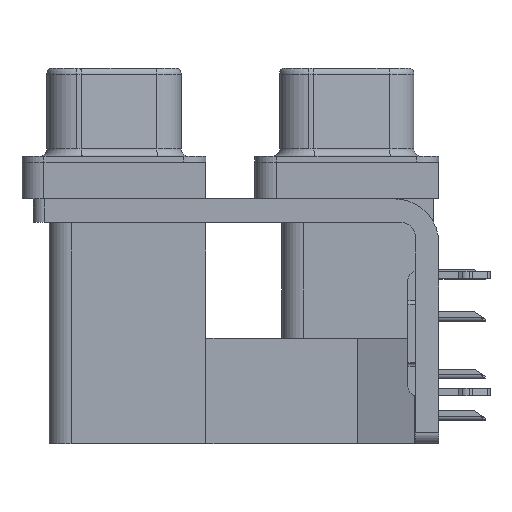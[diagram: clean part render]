
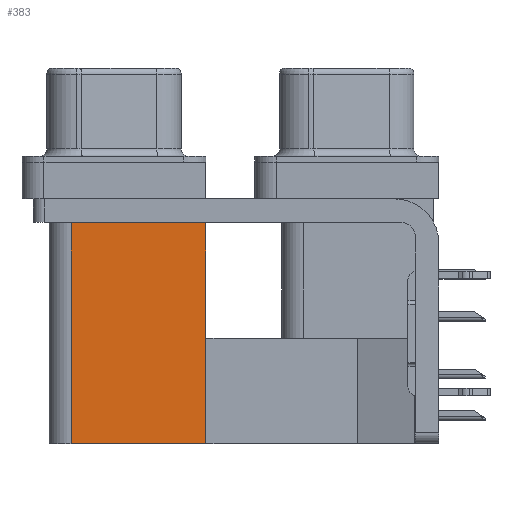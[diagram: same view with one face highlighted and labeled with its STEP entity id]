
A CAD part, left-side view. The second image highlights one B-rep face of the part: STEP entity #383.
In plain terms, the highlighted planar face has unit normal (-1, 0, 0).
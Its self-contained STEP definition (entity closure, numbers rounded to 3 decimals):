
#65 = AXIS2_PLACEMENT_3D ( 'NONE', #16014, #2208, #369 ) ;
#312 = VERTEX_POINT ( 'NONE', #13531 ) ;
#369 = DIRECTION ( 'NONE',  ( 0., 0., -1. ) ) ;
#383 = ADVANCED_FACE ( 'NONE', ( #8005 ), #22569, .F. ) ;
#1462 = LINE ( 'NONE', #24841, #5147 ) ;
#1758 = VECTOR ( 'NONE', #3354, 1000. ) ;
#1886 = EDGE_CURVE ( 'NONE', #18870, #14681, #2831, .T. ) ;
#2208 = DIRECTION ( 'NONE',  ( 1., 0., 0. ) ) ;
#2485 = VECTOR ( 'NONE', #20062, 1000. ) ;
#2831 = LINE ( 'NONE', #25289, #1758 ) ;
#3354 = DIRECTION ( 'NONE',  ( 0., 0., 1. ) ) ;
#4014 = ORIENTED_EDGE ( 'NONE', *, *, #1886, .T. ) ;
#4415 = EDGE_CURVE ( 'NONE', #18870, #7563, #24840, .T. ) ;
#5147 = VECTOR ( 'NONE', #17344, 1000. ) ;
#6847 = CARTESIAN_POINT ( 'NONE',  ( 3.79, 9.6, -19.2 ) ) ;
#7563 = VERTEX_POINT ( 'NONE', #13331 ) ;
#7720 = ORIENTED_EDGE ( 'NONE', *, *, #4415, .F. ) ;
#8005 = FACE_OUTER_BOUND ( 'NONE', #17991, .T. ) ;
#10920 = CARTESIAN_POINT ( 'NONE',  ( 3.79, 9.6, -2.5 ) ) ;
#11751 = ORIENTED_EDGE ( 'NONE', *, *, #19619, .T. ) ;
#13331 = CARTESIAN_POINT ( 'NONE',  ( 3.79, 18.8, -19.2 ) ) ;
#13531 = CARTESIAN_POINT ( 'NONE',  ( 3.79, 18.8, -2.5 ) ) ;
#14681 = VERTEX_POINT ( 'NONE', #10920 ) ;
#15312 = VECTOR ( 'NONE', #16956, 1000. ) ;
#16014 = CARTESIAN_POINT ( 'NONE',  ( 3.79, 9.6, -19.2 ) ) ;
#16956 = DIRECTION ( 'NONE',  ( 0., 1., 0. ) ) ;
#17344 = DIRECTION ( 'NONE',  ( 0., 0., 1. ) ) ;
#17991 = EDGE_LOOP ( 'NONE', ( #11751, #24680, #7720, #4014 ) ) ;
#18088 = CARTESIAN_POINT ( 'NONE',  ( 3.79, 9.6, -2.5 ) ) ;
#18870 = VERTEX_POINT ( 'NONE', #24719 ) ;
#19619 = EDGE_CURVE ( 'NONE', #14681, #312, #19804, .T. ) ;
#19804 = LINE ( 'NONE', #18088, #2485 ) ;
#20062 = DIRECTION ( 'NONE',  ( 0., 1., 0. ) ) ;
#22569 = PLANE ( 'NONE',  #65 ) ;
#23116 = EDGE_CURVE ( 'NONE', #7563, #312, #1462, .T. ) ;
#24680 = ORIENTED_EDGE ( 'NONE', *, *, #23116, .F. ) ;
#24719 = CARTESIAN_POINT ( 'NONE',  ( 3.79, 9.6, -19.2 ) ) ;
#24840 = LINE ( 'NONE', #6847, #15312 ) ;
#24841 = CARTESIAN_POINT ( 'NONE',  ( 3.79, 18.8, -19.2 ) ) ;
#25289 = CARTESIAN_POINT ( 'NONE',  ( 3.79, 9.6, -19.2 ) ) ;
